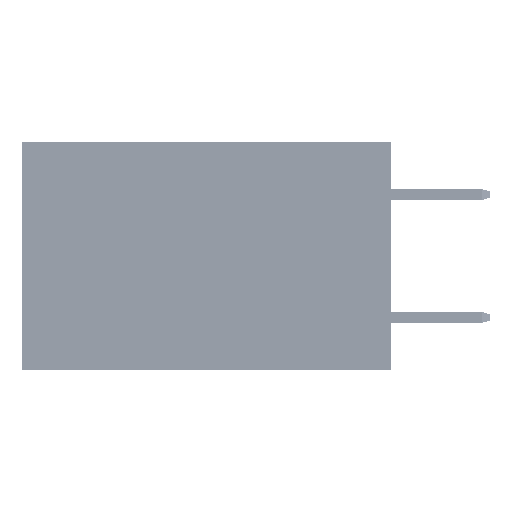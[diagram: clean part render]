
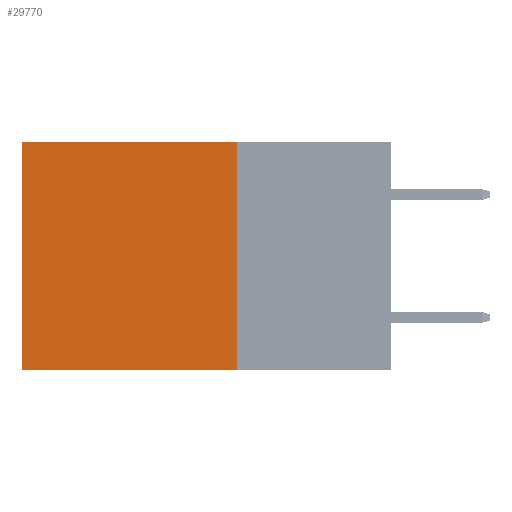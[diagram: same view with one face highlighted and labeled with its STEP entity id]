
A CAD part, left-side view. The second image highlights one B-rep face of the part: STEP entity #29770.
In plain terms, the highlighted planar face has unit normal (-1, 0, 0).
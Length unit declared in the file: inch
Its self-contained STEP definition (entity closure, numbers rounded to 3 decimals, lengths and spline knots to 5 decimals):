
#5051 = EDGE_CURVE ( 'NONE', #25096, #36927, #46542, .T. ) ;
#6368 = EDGE_CURVE ( 'NONE', #7367, #36927, #36034, .T. ) ;
#6540 = LINE ( 'NONE', #35750, #38922 ) ;
#7197 = CARTESIAN_POINT ( 'NONE',  ( 0.2875, 0.25, 0. ) ) ;
#7367 = VERTEX_POINT ( 'NONE', #18474 ) ;
#8561 = ORIENTED_EDGE ( 'NONE', *, *, #5051, .T. ) ;
#8839 = CARTESIAN_POINT ( 'NONE',  ( 0.2875, 0.25, 0. ) ) ;
#9306 = CARTESIAN_POINT ( 'NONE',  ( 0.2875, 0.6, 0. ) ) ;
#12509 = CARTESIAN_POINT ( 'NONE',  ( 0.2875, 0.6, 0. ) ) ;
#13002 = VECTOR ( 'NONE', #38704, 39.37008 ) ;
#14190 = PLANE ( 'NONE',  #40010 ) ;
#18474 = CARTESIAN_POINT ( 'NONE',  ( 0.2875, 0.25, -0.37 ) ) ;
#20867 = DIRECTION ( 'NONE',  ( 0., 1., 0. ) ) ;
#21959 = EDGE_CURVE ( 'NONE', #40782, #25096, #6540, .T. ) ;
#22069 = EDGE_LOOP ( 'NONE', ( #8561, #26813, #25312, #46760 ) ) ;
#24285 = CARTESIAN_POINT ( 'NONE',  ( 0.2875, 0.6, -0.37 ) ) ;
#25096 = VERTEX_POINT ( 'NONE', #9306 ) ;
#25312 = ORIENTED_EDGE ( 'NONE', *, *, #33281, .F. ) ;
#26813 = ORIENTED_EDGE ( 'NONE', *, *, #6368, .F. ) ;
#27419 = DIRECTION ( 'NONE',  ( 0., 0., -1. ) ) ;
#28891 = DIRECTION ( 'NONE',  ( 0., 0., -1. ) ) ;
#29770 = ADVANCED_FACE ( 'NONE', ( #41144 ), #14190, .F. ) ;
#31372 = VECTOR ( 'NONE', #47007, 39.37008 ) ;
#33281 = EDGE_CURVE ( 'NONE', #40782, #7367, #40776, .T. ) ;
#35750 = CARTESIAN_POINT ( 'NONE',  ( 0.2875, 0.25, 0. ) ) ;
#36034 = LINE ( 'NONE', #43123, #31372 ) ;
#36927 = VERTEX_POINT ( 'NONE', #24285 ) ;
#38451 = VECTOR ( 'NONE', #27419, 39.37008 ) ;
#38704 = DIRECTION ( 'NONE',  ( 0., 0., -1. ) ) ;
#38922 = VECTOR ( 'NONE', #20867, 39.37008 ) ;
#40010 = AXIS2_PLACEMENT_3D ( 'NONE', #43770, #47662, #28891 ) ;
#40776 = LINE ( 'NONE', #8839, #38451 ) ;
#40782 = VERTEX_POINT ( 'NONE', #7197 ) ;
#41144 = FACE_OUTER_BOUND ( 'NONE', #22069, .T. ) ;
#43123 = CARTESIAN_POINT ( 'NONE',  ( 0.2875, 0.25, -0.37 ) ) ;
#43770 = CARTESIAN_POINT ( 'NONE',  ( 0.2875, 0.25, 0. ) ) ;
#46542 = LINE ( 'NONE', #12509, #13002 ) ;
#46760 = ORIENTED_EDGE ( 'NONE', *, *, #21959, .T. ) ;
#47007 = DIRECTION ( 'NONE',  ( 0., 1., 0. ) ) ;
#47662 = DIRECTION ( 'NONE',  ( 1., 0., 0. ) ) ;
